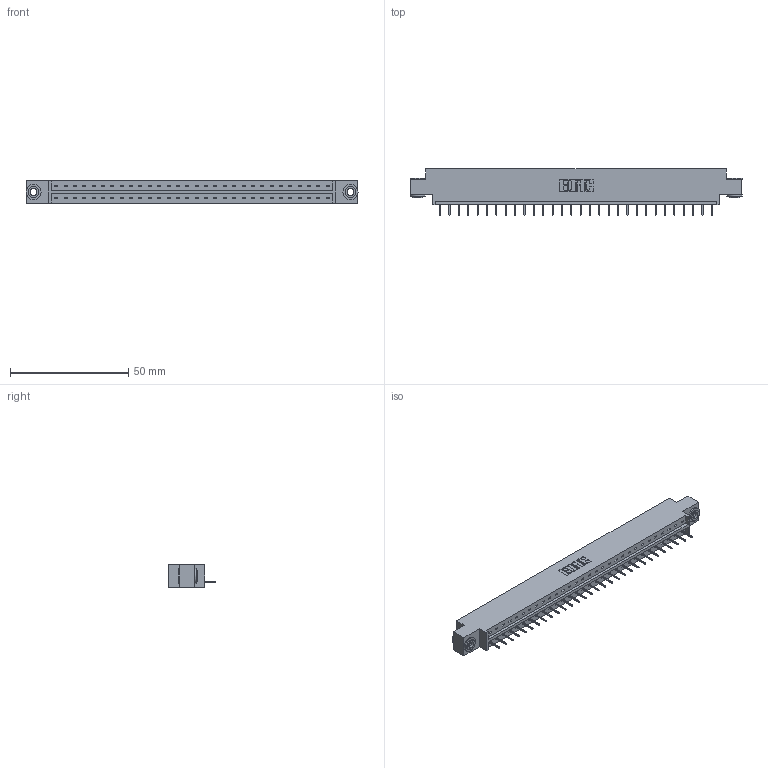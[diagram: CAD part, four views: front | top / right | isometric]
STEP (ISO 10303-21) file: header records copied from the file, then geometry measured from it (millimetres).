
FILE_DESCRIPTION (( 'STEP AP203' ), '1' );
FILE_NAME ('333-030-524-603.STEP', '2018-08-02T17:41:14', ( '' ), ( '' ), 'SwSTEP 2.0', 'SolidWorks 2016', '' );
FILE_SCHEMA (( 'CONFIG_CONTROL_DESIGN' ));
Length unit declared in the file: inch
Products named in the file (4): 333 Part_Offset - .156 Dia - TH; 345-292-001_345-293-124; 345-250-002_345-250-002-102; 333-030-524-603
Assembly tree (33 placements, depth 2):
  333-030-524-603
    333 Part_Offset - .156 Dia - TH
    345-292-001_345-293-124  x30
    345-250-002_345-250-002-102  x2
Bounding box: 140.41 x 19.69 x 9.4 mm (x, y, z)
Volume: 13699.2 mm3; surface area: 14762.1 mm2
Topology: 33 solids, 33 shells, 2016 faces, 5799 edges, 3742 vertices
Faces by surface type: plane 1524, cylinder 484, cone 8
Entity records: 20748 total; most frequent: CARTESIAN_POINT 3559, ORIENTED_EDGE 3518, DIRECTION 3061, EDGE_CURVE 1759, VECTOR 1611, LINE 1611, VERTEX_POINT 1166, AXIS2_PLACEMENT_3D 725
